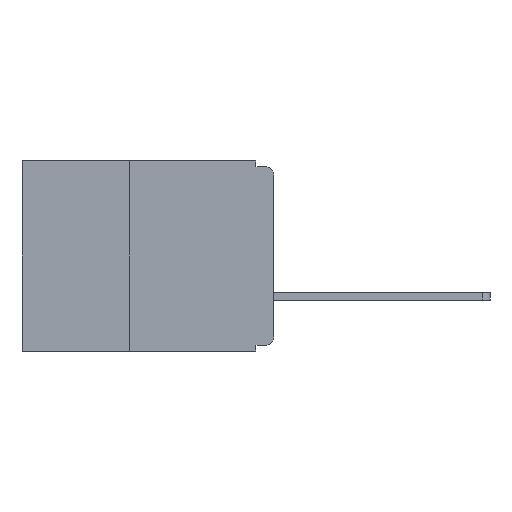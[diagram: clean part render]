
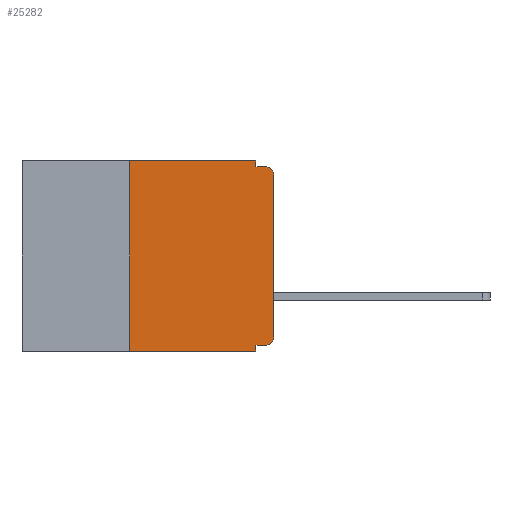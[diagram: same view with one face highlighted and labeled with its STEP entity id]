
A CAD part, left-side view. The second image highlights one B-rep face of the part: STEP entity #25282.
In plain terms, the highlighted planar face has unit normal (-1, 0, 0).
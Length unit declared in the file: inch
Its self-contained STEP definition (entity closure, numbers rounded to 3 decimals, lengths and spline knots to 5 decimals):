
#284 = LINE ( 'NONE', #21259, #27602 ) ;
#524 = VERTEX_POINT ( 'NONE', #24900 ) ;
#689 = EDGE_CURVE ( 'NONE', #3642, #28192, #32780, .T. ) ;
#702 = CIRCLE ( 'NONE', #31134, 0.015 ) ;
#975 = VECTOR ( 'NONE', #13095, 39.37008 ) ;
#1153 = FACE_OUTER_BOUND ( 'NONE', #26381, .T. ) ;
#1364 = EDGE_CURVE ( 'NONE', #524, #9863, #32327, .T. ) ;
#1719 = DIRECTION ( 'NONE',  ( 0., 1., 0. ) ) ;
#2542 = CARTESIAN_POINT ( 'NONE',  ( 0., 0.031, -0.33 ) ) ;
#3566 = ORIENTED_EDGE ( 'NONE', *, *, #26845, .F. ) ;
#3642 = VERTEX_POINT ( 'NONE', #4522 ) ;
#3696 = ORIENTED_EDGE ( 'NONE', *, *, #27405, .F. ) ;
#3931 = CARTESIAN_POINT ( 'NONE',  ( 0., 0.031, 0. ) ) ;
#4522 = CARTESIAN_POINT ( 'NONE',  ( 0., 0.031, -0.32 ) ) ;
#5042 = EDGE_CURVE ( 'NONE', #23882, #33568, #284, .T. ) ;
#5083 = VECTOR ( 'NONE', #21859, 39.37008 ) ;
#5185 = DIRECTION ( 'NONE',  ( 0., -1., 0. ) ) ;
#5397 = CARTESIAN_POINT ( 'NONE',  ( 0., 0.015, -0.025 ) ) ;
#5584 = CARTESIAN_POINT ( 'NONE',  ( 0., 0., -0.305 ) ) ;
#7325 = LINE ( 'NONE', #21071, #8151 ) ;
#8041 = DIRECTION ( 'NONE',  ( 0., -1., 0. ) ) ;
#8049 = DIRECTION ( 'NONE',  ( 0., 0., -1. ) ) ;
#8151 = VECTOR ( 'NONE', #5185, 39.37008 ) ;
#9056 = VERTEX_POINT ( 'NONE', #21358 ) ;
#9593 = CARTESIAN_POINT ( 'NONE',  ( 0., 0., -0.32 ) ) ;
#9863 = VERTEX_POINT ( 'NONE', #25643 ) ;
#9891 = DIRECTION ( 'NONE',  ( 0., 0., 1. ) ) ;
#10064 = VECTOR ( 'NONE', #9891, 39.37008 ) ;
#10916 = DIRECTION ( 'NONE',  ( 0., 0., 1. ) ) ;
#11296 = CARTESIAN_POINT ( 'NONE',  ( 0., 0.015, -0.305 ) ) ;
#12314 = PLANE ( 'NONE',  #25766 ) ;
#13058 = EDGE_CURVE ( 'NONE', #33568, #15504, #702, .T. ) ;
#13095 = DIRECTION ( 'NONE',  ( 0., -1., 0. ) ) ;
#13246 = VERTEX_POINT ( 'NONE', #14518 ) ;
#13968 = DIRECTION ( 'NONE',  ( 0., 0., -1. ) ) ;
#14518 = CARTESIAN_POINT ( 'NONE',  ( 0., 0.015, -0.32 ) ) ;
#14779 = CARTESIAN_POINT ( 'NONE',  ( 0., 0.015, -0.01 ) ) ;
#14991 = CARTESIAN_POINT ( 'NONE',  ( 0., 0.437, 0. ) ) ;
#15504 = VERTEX_POINT ( 'NONE', #14779 ) ;
#15596 = EDGE_CURVE ( 'NONE', #31534, #9056, #17113, .T. ) ;
#15713 = CARTESIAN_POINT ( 'NONE',  ( 0., 0., -0.025 ) ) ;
#15944 = LINE ( 'NONE', #23754, #975 ) ;
#16247 = ORIENTED_EDGE ( 'NONE', *, *, #5042, .T. ) ;
#17113 = LINE ( 'NONE', #23106, #10064 ) ;
#17356 = VECTOR ( 'NONE', #1719, 39.37008 ) ;
#17622 = DIRECTION ( 'NONE',  ( 0., 0., -1. ) ) ;
#18584 = CARTESIAN_POINT ( 'NONE',  ( 0., 0.437, 0. ) ) ;
#20260 = ORIENTED_EDGE ( 'NONE', *, *, #30752, .T. ) ;
#21071 = CARTESIAN_POINT ( 'NONE',  ( 0., 0.437, -0.33 ) ) ;
#21259 = CARTESIAN_POINT ( 'NONE',  ( 0., 0., 0. ) ) ;
#21358 = CARTESIAN_POINT ( 'NONE',  ( 0., 0.25, 0. ) ) ;
#21565 = ORIENTED_EDGE ( 'NONE', *, *, #13058, .T. ) ;
#21859 = DIRECTION ( 'NONE',  ( 0., 0., -1. ) ) ;
#22363 = CARTESIAN_POINT ( 'NONE',  ( 0., 0.25, -0.33 ) ) ;
#22579 = EDGE_CURVE ( 'NONE', #13246, #3642, #24408, .T. ) ;
#23106 = CARTESIAN_POINT ( 'NONE',  ( 0., 0.25, -0.33 ) ) ;
#23754 = CARTESIAN_POINT ( 'NONE',  ( 0., 0., -0.01 ) ) ;
#23882 = VERTEX_POINT ( 'NONE', #5584 ) ;
#23927 = DIRECTION ( 'NONE',  ( -1., 0., 0. ) ) ;
#24408 = LINE ( 'NONE', #9593, #17356 ) ;
#24900 = CARTESIAN_POINT ( 'NONE',  ( 0., 0.031, 0. ) ) ;
#25282 = ADVANCED_FACE ( 'NONE', ( #1153 ), #12314, .F. ) ;
#25643 = CARTESIAN_POINT ( 'NONE',  ( 0., 0.031, -0.01 ) ) ;
#25766 = AXIS2_PLACEMENT_3D ( 'NONE', #14991, #33374, #17622 ) ;
#25839 = VECTOR ( 'NONE', #30660, 39.37008 ) ;
#26217 = EDGE_CURVE ( 'NONE', #31534, #28192, #7325, .T. ) ;
#26297 = AXIS2_PLACEMENT_3D ( 'NONE', #11296, #29776, #13968 ) ;
#26302 = VECTOR ( 'NONE', #8041, 39.37008 ) ;
#26381 = EDGE_LOOP ( 'NONE', ( #16247, #21565, #3696, #28842, #3566, #28980, #29460, #34042, #28373, #20260 ) ) ;
#26845 = EDGE_CURVE ( 'NONE', #9056, #524, #28773, .T. ) ;
#27405 = EDGE_CURVE ( 'NONE', #9863, #15504, #15944, .T. ) ;
#27602 = VECTOR ( 'NONE', #10916, 39.37008 ) ;
#28133 = CIRCLE ( 'NONE', #26297, 0.015 ) ;
#28192 = VERTEX_POINT ( 'NONE', #29897 ) ;
#28373 = ORIENTED_EDGE ( 'NONE', *, *, #22579, .F. ) ;
#28773 = LINE ( 'NONE', #18584, #26302 ) ;
#28842 = ORIENTED_EDGE ( 'NONE', *, *, #1364, .F. ) ;
#28980 = ORIENTED_EDGE ( 'NONE', *, *, #15596, .F. ) ;
#29460 = ORIENTED_EDGE ( 'NONE', *, *, #26217, .T. ) ;
#29776 = DIRECTION ( 'NONE',  ( -1., 0., 0. ) ) ;
#29897 = CARTESIAN_POINT ( 'NONE',  ( 0., 0.031, -0.33 ) ) ;
#30660 = DIRECTION ( 'NONE',  ( 0., 0., -1. ) ) ;
#30752 = EDGE_CURVE ( 'NONE', #13246, #23882, #28133, .T. ) ;
#31134 = AXIS2_PLACEMENT_3D ( 'NONE', #5397, #23927, #8049 ) ;
#31534 = VERTEX_POINT ( 'NONE', #22363 ) ;
#32327 = LINE ( 'NONE', #3931, #5083 ) ;
#32780 = LINE ( 'NONE', #2542, #25839 ) ;
#33374 = DIRECTION ( 'NONE',  ( 1., 0., 0. ) ) ;
#33568 = VERTEX_POINT ( 'NONE', #15713 ) ;
#34042 = ORIENTED_EDGE ( 'NONE', *, *, #689, .F. ) ;
